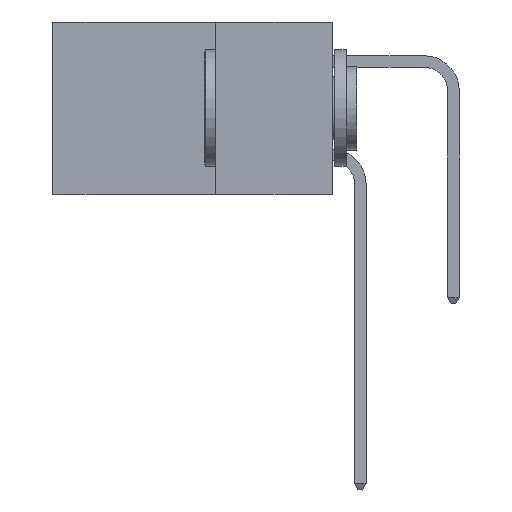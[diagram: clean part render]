
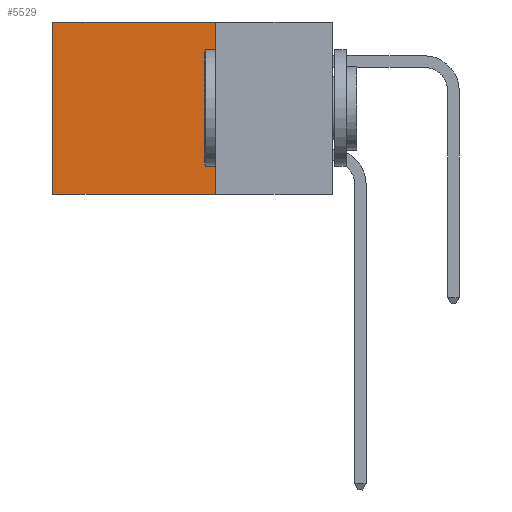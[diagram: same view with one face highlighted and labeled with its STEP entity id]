
A CAD part, left-side view. The second image highlights one B-rep face of the part: STEP entity #5529.
In plain terms, the highlighted planar face has unit normal (-1, 0, 0).
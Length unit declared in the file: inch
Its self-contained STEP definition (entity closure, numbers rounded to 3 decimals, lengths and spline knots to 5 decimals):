
#303 = CARTESIAN_POINT ( 'NONE',  ( 0.298, 0.25, 0. ) ) ;
#314 = DIRECTION ( 'NONE',  ( 0., 1., 0. ) ) ;
#317 = VECTOR ( 'NONE', #8426, 39.37008 ) ;
#871 = DIRECTION ( 'NONE',  ( 1., 0., 0. ) ) ;
#1345 = EDGE_LOOP ( 'NONE', ( #8673, #7407, #9907, #10733 ) ) ;
#1469 = CARTESIAN_POINT ( 'NONE',  ( 0.298, 0.25, 0. ) ) ;
#2404 = VERTEX_POINT ( 'NONE', #6005 ) ;
#2609 = VERTEX_POINT ( 'NONE', #1469 ) ;
#3195 = AXIS2_PLACEMENT_3D ( 'NONE', #5775, #871, #7988 ) ;
#3337 = VECTOR ( 'NONE', #314, 39.37008 ) ;
#3840 = CARTESIAN_POINT ( 'NONE',  ( 0.298, 0.6, 0. ) ) ;
#3864 = VECTOR ( 'NONE', #9864, 39.37008 ) ;
#4558 = VERTEX_POINT ( 'NONE', #11379 ) ;
#4868 = VERTEX_POINT ( 'NONE', #11237 ) ;
#5195 = EDGE_CURVE ( 'NONE', #2609, #4868, #11490, .T. ) ;
#5529 = ADVANCED_FACE ( 'NONE', ( #5683 ), #8965, .F. ) ;
#5683 = FACE_OUTER_BOUND ( 'NONE', #1345, .T. ) ;
#5775 = CARTESIAN_POINT ( 'NONE',  ( 0.298, 0.25, 0. ) ) ;
#5796 = EDGE_CURVE ( 'NONE', #2609, #4558, #10471, .T. ) ;
#6005 = CARTESIAN_POINT ( 'NONE',  ( 0.298, 0.6, -0.37 ) ) ;
#6313 = DIRECTION ( 'NONE',  ( 0., 1., 0. ) ) ;
#7047 = EDGE_CURVE ( 'NONE', #4558, #2404, #11381, .T. ) ;
#7407 = ORIENTED_EDGE ( 'NONE', *, *, #7047, .F. ) ;
#7988 = DIRECTION ( 'NONE',  ( 0., 0., -1. ) ) ;
#8426 = DIRECTION ( 'NONE',  ( 0., 0., -1. ) ) ;
#8673 = ORIENTED_EDGE ( 'NONE', *, *, #11295, .T. ) ;
#8811 = VECTOR ( 'NONE', #6313, 39.37008 ) ;
#8965 = PLANE ( 'NONE',  #3195 ) ;
#9225 = LINE ( 'NONE', #3840, #3864 ) ;
#9864 = DIRECTION ( 'NONE',  ( 0., 0., -1. ) ) ;
#9907 = ORIENTED_EDGE ( 'NONE', *, *, #5796, .F. ) ;
#10471 = LINE ( 'NONE', #303, #317 ) ;
#10733 = ORIENTED_EDGE ( 'NONE', *, *, #5195, .T. ) ;
#11237 = CARTESIAN_POINT ( 'NONE',  ( 0.298, 0.6, 0. ) ) ;
#11295 = EDGE_CURVE ( 'NONE', #4868, #2404, #9225, .T. ) ;
#11304 = CARTESIAN_POINT ( 'NONE',  ( 0.298, 0.25, 0. ) ) ;
#11356 = CARTESIAN_POINT ( 'NONE',  ( 0.298, 0.25, -0.37 ) ) ;
#11379 = CARTESIAN_POINT ( 'NONE',  ( 0.298, 0.25, -0.37 ) ) ;
#11381 = LINE ( 'NONE', #11356, #3337 ) ;
#11490 = LINE ( 'NONE', #11304, #8811 ) ;
